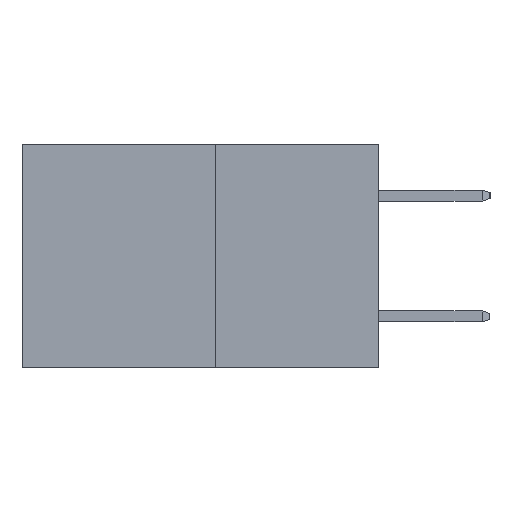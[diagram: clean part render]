
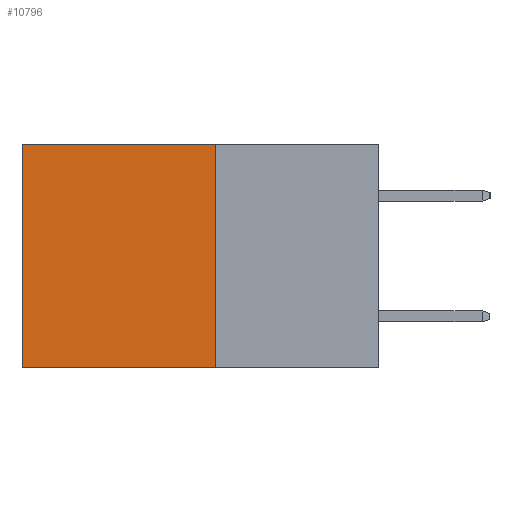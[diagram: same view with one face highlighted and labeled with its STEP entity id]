
A CAD part, left-side view. The second image highlights one B-rep face of the part: STEP entity #10796.
In plain terms, the highlighted planar face has unit normal (-1, 0, 0).
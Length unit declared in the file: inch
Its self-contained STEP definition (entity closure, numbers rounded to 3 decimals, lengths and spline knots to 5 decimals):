
#103 = VERTEX_POINT ( 'NONE', #5414 ) ;
#191 = CARTESIAN_POINT ( 'NONE',  ( 0.277, 0.27, -0.37 ) ) ;
#193 = LINE ( 'NONE', #10639, #2488 ) ;
#1752 = DIRECTION ( 'NONE',  ( 0., 1., 0. ) ) ;
#1915 = DIRECTION ( 'NONE',  ( 1., 0., 0. ) ) ;
#2147 = VERTEX_POINT ( 'NONE', #191 ) ;
#2488 = VECTOR ( 'NONE', #2904, 39.37008 ) ;
#2904 = DIRECTION ( 'NONE',  ( 0., 0., -1. ) ) ;
#2907 = CARTESIAN_POINT ( 'NONE',  ( 0.277, 0.27, -0.37 ) ) ;
#3456 = EDGE_LOOP ( 'NONE', ( #9341, #8581, #9034, #7123 ) ) ;
#3478 = LINE ( 'NONE', #3518, #7757 ) ;
#3518 = CARTESIAN_POINT ( 'NONE',  ( 0.277, 0.27, 0. ) ) ;
#4383 = EDGE_CURVE ( 'NONE', #2147, #103, #4909, .T. ) ;
#4864 = CARTESIAN_POINT ( 'NONE',  ( 0.277, 0.27, 0. ) ) ;
#4909 = LINE ( 'NONE', #8224, #9764 ) ;
#5232 = EDGE_CURVE ( 'NONE', #9283, #8288, #3478, .T. ) ;
#5414 = CARTESIAN_POINT ( 'NONE',  ( 0.277, 0.59, -0.37 ) ) ;
#6339 = FACE_OUTER_BOUND ( 'NONE', #3456, .T. ) ;
#6570 = EDGE_CURVE ( 'NONE', #8288, #103, #193, .T. ) ;
#7123 = ORIENTED_EDGE ( 'NONE', *, *, #5232, .T. ) ;
#7757 = VECTOR ( 'NONE', #1752, 39.37008 ) ;
#7798 = PLANE ( 'NONE',  #10648 ) ;
#8208 = DIRECTION ( 'NONE',  ( 0., 1., 0. ) ) ;
#8224 = CARTESIAN_POINT ( 'NONE',  ( 0.277, 0.27, -0.37 ) ) ;
#8288 = VERTEX_POINT ( 'NONE', #11963 ) ;
#8530 = VECTOR ( 'NONE', #10694, 39.37008 ) ;
#8581 = ORIENTED_EDGE ( 'NONE', *, *, #4383, .F. ) ;
#8781 = EDGE_CURVE ( 'NONE', #9283, #2147, #11067, .T. ) ;
#8794 = DIRECTION ( 'NONE',  ( 0., 0., -1. ) ) ;
#9034 = ORIENTED_EDGE ( 'NONE', *, *, #8781, .F. ) ;
#9283 = VERTEX_POINT ( 'NONE', #4864 ) ;
#9341 = ORIENTED_EDGE ( 'NONE', *, *, #6570, .T. ) ;
#9717 = CARTESIAN_POINT ( 'NONE',  ( 0.277, 0.27, -0.37 ) ) ;
#9764 = VECTOR ( 'NONE', #8208, 39.37008 ) ;
#10639 = CARTESIAN_POINT ( 'NONE',  ( 0.277, 0.59, -0.37 ) ) ;
#10648 = AXIS2_PLACEMENT_3D ( 'NONE', #9717, #1915, #8794 ) ;
#10694 = DIRECTION ( 'NONE',  ( 0., 0., -1. ) ) ;
#10796 = ADVANCED_FACE ( 'NONE', ( #6339 ), #7798, .F. ) ;
#11067 = LINE ( 'NONE', #2907, #8530 ) ;
#11963 = CARTESIAN_POINT ( 'NONE',  ( 0.277, 0.59, 0. ) ) ;
